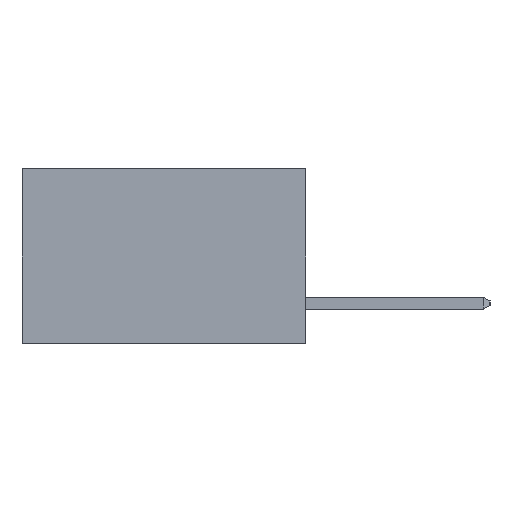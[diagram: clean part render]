
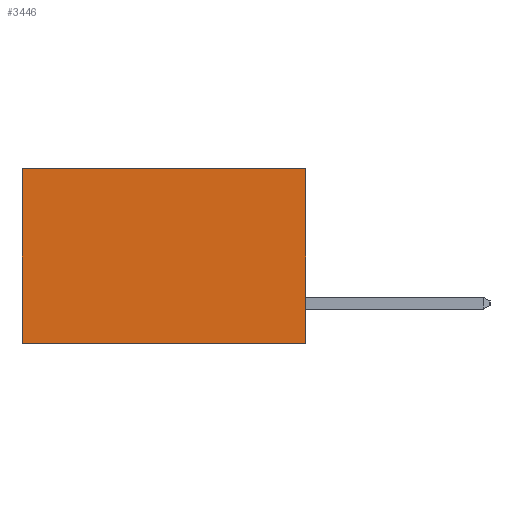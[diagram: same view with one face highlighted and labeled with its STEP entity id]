
A CAD part, left-side view. The second image highlights one B-rep face of the part: STEP entity #3446.
In plain terms, the highlighted planar face has unit normal (-1, 0, 0).
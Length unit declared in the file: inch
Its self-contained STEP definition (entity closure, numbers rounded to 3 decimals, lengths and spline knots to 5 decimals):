
#528 = LINE ( 'NONE', #9263, #15332 ) ;
#851 = ORIENTED_EDGE ( 'NONE', *, *, #4911, .F. ) ;
#1468 = VERTEX_POINT ( 'NONE', #18576 ) ;
#1764 = VERTEX_POINT ( 'NONE', #6178 ) ;
#1794 = EDGE_CURVE ( 'NONE', #1468, #16936, #7115, .T. ) ;
#1885 = VECTOR ( 'NONE', #22615, 39.37008 ) ;
#3446 = ADVANCED_FACE ( 'NONE', ( #14419 ), #9484, .F. ) ;
#3678 = EDGE_LOOP ( 'NONE', ( #17899, #11511, #851, #5719 ) ) ;
#4911 = EDGE_CURVE ( 'NONE', #16624, #1468, #11729, .T. ) ;
#5719 = ORIENTED_EDGE ( 'NONE', *, *, #8861, .T. ) ;
#6178 = CARTESIAN_POINT ( 'NONE',  ( 0.2615, 0.6, 0. ) ) ;
#6681 = VECTOR ( 'NONE', #18565, 39.37008 ) ;
#7115 = LINE ( 'NONE', #14028, #1885 ) ;
#7988 = VECTOR ( 'NONE', #19267, 39.37008 ) ;
#8861 = EDGE_CURVE ( 'NONE', #16624, #1764, #22862, .T. ) ;
#9263 = CARTESIAN_POINT ( 'NONE',  ( 0.2615, 0.6, -0.37 ) ) ;
#9461 = DIRECTION ( 'NONE',  ( 1., 0., 0. ) ) ;
#9484 = PLANE ( 'NONE',  #10353 ) ;
#9491 = CARTESIAN_POINT ( 'NONE',  ( 0.2615, 0., -0.37 ) ) ;
#9562 = DIRECTION ( 'NONE',  ( 0., 0., -1. ) ) ;
#9973 = DIRECTION ( 'NONE',  ( 0., 0., -1. ) ) ;
#10027 = EDGE_CURVE ( 'NONE', #1764, #16936, #528, .T. ) ;
#10353 = AXIS2_PLACEMENT_3D ( 'NONE', #9491, #9461, #9562 ) ;
#10425 = CARTESIAN_POINT ( 'NONE',  ( 0.2615, 0., 0. ) ) ;
#11279 = CARTESIAN_POINT ( 'NONE',  ( 0.2615, 0.6, -0.37 ) ) ;
#11511 = ORIENTED_EDGE ( 'NONE', *, *, #1794, .F. ) ;
#11729 = LINE ( 'NONE', #19525, #6681 ) ;
#14028 = CARTESIAN_POINT ( 'NONE',  ( 0.2615, 0., -0.37 ) ) ;
#14419 = FACE_OUTER_BOUND ( 'NONE', #3678, .T. ) ;
#15332 = VECTOR ( 'NONE', #9973, 39.37008 ) ;
#16161 = CARTESIAN_POINT ( 'NONE',  ( 0.2615, 0., 0. ) ) ;
#16624 = VERTEX_POINT ( 'NONE', #10425 ) ;
#16936 = VERTEX_POINT ( 'NONE', #11279 ) ;
#17899 = ORIENTED_EDGE ( 'NONE', *, *, #10027, .T. ) ;
#18565 = DIRECTION ( 'NONE',  ( 0., 0., -1. ) ) ;
#18576 = CARTESIAN_POINT ( 'NONE',  ( 0.2615, 0., -0.37 ) ) ;
#19267 = DIRECTION ( 'NONE',  ( 0., 1., 0. ) ) ;
#19525 = CARTESIAN_POINT ( 'NONE',  ( 0.2615, 0., -0.37 ) ) ;
#22615 = DIRECTION ( 'NONE',  ( 0., 1., 0. ) ) ;
#22862 = LINE ( 'NONE', #16161, #7988 ) ;
